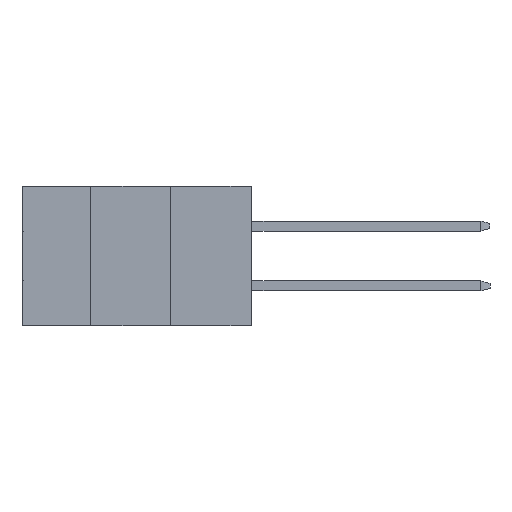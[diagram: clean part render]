
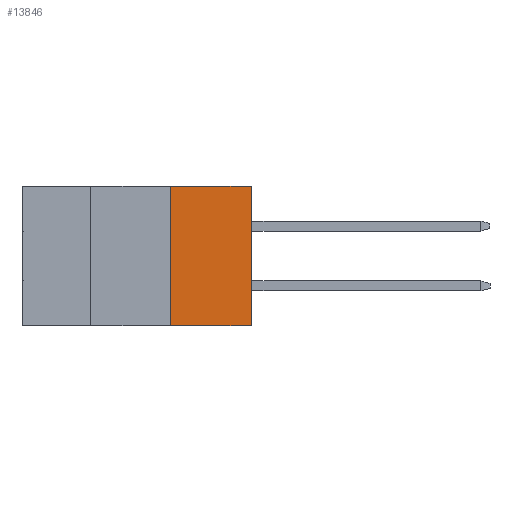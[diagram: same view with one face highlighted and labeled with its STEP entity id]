
A CAD part, left-side view. The second image highlights one B-rep face of the part: STEP entity #13846.
In plain terms, the highlighted planar face has unit normal (-1, 0, 0).
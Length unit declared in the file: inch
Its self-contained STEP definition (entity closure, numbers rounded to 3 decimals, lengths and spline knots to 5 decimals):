
#840 = LINE ( 'NONE', #20978, #10591 ) ;
#906 = VERTEX_POINT ( 'NONE', #6650 ) ;
#1041 = EDGE_CURVE ( 'NONE', #11187, #21551, #3421, .T. ) ;
#1699 = CARTESIAN_POINT ( 'NONE',  ( 0.4265, 0., -0.437 ) ) ;
#3421 = LINE ( 'NONE', #21784, #15660 ) ;
#3768 = DIRECTION ( 'NONE',  ( 0., 0., 1. ) ) ;
#5431 = DIRECTION ( 'NONE',  ( 0., 0., -1. ) ) ;
#5939 = CARTESIAN_POINT ( 'NONE',  ( 0.4265, 0.254, 0. ) ) ;
#6650 = CARTESIAN_POINT ( 'NONE',  ( 0.4265, 0., -0.437 ) ) ;
#7228 = VERTEX_POINT ( 'NONE', #12800 ) ;
#7932 = VECTOR ( 'NONE', #18059, 39.37008 ) ;
#8930 = DIRECTION ( 'NONE',  ( 0., 0., 1. ) ) ;
#8989 = CARTESIAN_POINT ( 'NONE',  ( 0.4265, 0.254, -0.437 ) ) ;
#9224 = FACE_OUTER_BOUND ( 'NONE', #23175, .T. ) ;
#9924 = EDGE_CURVE ( 'NONE', #906, #7228, #21499, .T. ) ;
#10415 = AXIS2_PLACEMENT_3D ( 'NONE', #8989, #20123, #5431 ) ;
#10591 = VECTOR ( 'NONE', #18962, 39.37008 ) ;
#11187 = VERTEX_POINT ( 'NONE', #17735 ) ;
#12533 = ORIENTED_EDGE ( 'NONE', *, *, #19760, .F. ) ;
#12800 = CARTESIAN_POINT ( 'NONE',  ( 0.4265, 0., 0. ) ) ;
#13846 = ADVANCED_FACE ( 'NONE', ( #9224 ), #17992, .F. ) ;
#15660 = VECTOR ( 'NONE', #3768, 39.37008 ) ;
#16712 = ORIENTED_EDGE ( 'NONE', *, *, #9924, .T. ) ;
#17151 = ORIENTED_EDGE ( 'NONE', *, *, #20378, .T. ) ;
#17227 = ORIENTED_EDGE ( 'NONE', *, *, #1041, .F. ) ;
#17735 = CARTESIAN_POINT ( 'NONE',  ( 0.4265, 0.254, -0.437 ) ) ;
#17992 = PLANE ( 'NONE',  #10415 ) ;
#18059 = DIRECTION ( 'NONE',  ( 0., -1., 0. ) ) ;
#18186 = LINE ( 'NONE', #20188, #7932 ) ;
#18962 = DIRECTION ( 'NONE',  ( 0., -1., 0. ) ) ;
#19760 = EDGE_CURVE ( 'NONE', #21551, #7228, #18186, .T. ) ;
#20123 = DIRECTION ( 'NONE',  ( 1., 0., 0. ) ) ;
#20188 = CARTESIAN_POINT ( 'NONE',  ( 0.4265, 0.254, 0. ) ) ;
#20378 = EDGE_CURVE ( 'NONE', #11187, #906, #840, .T. ) ;
#20978 = CARTESIAN_POINT ( 'NONE',  ( 0.4265, 0.254, -0.437 ) ) ;
#21499 = LINE ( 'NONE', #1699, #22643 ) ;
#21551 = VERTEX_POINT ( 'NONE', #5939 ) ;
#21784 = CARTESIAN_POINT ( 'NONE',  ( 0.4265, 0.254, -0.437 ) ) ;
#22643 = VECTOR ( 'NONE', #8930, 39.37008 ) ;
#23175 = EDGE_LOOP ( 'NONE', ( #16712, #12533, #17227, #17151 ) ) ;
